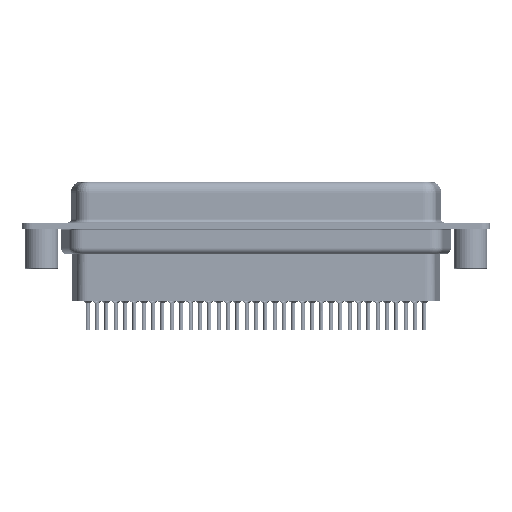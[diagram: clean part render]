
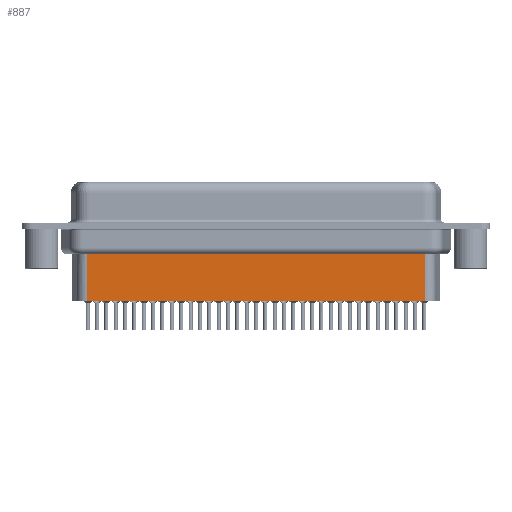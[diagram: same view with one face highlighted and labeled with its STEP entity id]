
A CAD part, front view. The second image highlights one B-rep face of the part: STEP entity #887.
In plain terms, the highlighted planar face has unit normal (0, -1, 0).
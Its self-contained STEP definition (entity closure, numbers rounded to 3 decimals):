
#887 = ADVANCED_FACE ( 'NONE', ( #9429 ), #2187, .T. ) ;
#2187 = PLANE ( 'NONE',  #17542 ) ;
#3297 = EDGE_CURVE ( 'NONE', #29896, #18458, #24506, .T. ) ;
#3354 = ORIENTED_EDGE ( 'NONE', *, *, #29043, .F. ) ;
#4019 = LINE ( 'NONE', #24741, #19696 ) ;
#4256 = ORIENTED_EDGE ( 'NONE', *, *, #20402, .F. ) ;
#4476 = DIRECTION ( 'NONE',  ( 0., 0., -1. ) ) ;
#6446 = CARTESIAN_POINT ( 'NONE',  ( 56.794, -3.5, -11.15 ) ) ;
#9429 = FACE_OUTER_BOUND ( 'NONE', #20702, .T. ) ;
#9587 = DIRECTION ( 'NONE',  ( -1., 0., 0. ) ) ;
#11562 = VECTOR ( 'NONE', #18019, 1000. ) ;
#11949 = DIRECTION ( 'NONE',  ( 0., -1., 0. ) ) ;
#13086 = CARTESIAN_POINT ( 'NONE',  ( 6.706, -3.5, -3.1 ) ) ;
#14567 = LINE ( 'NONE', #24340, #27772 ) ;
#15309 = ORIENTED_EDGE ( 'NONE', *, *, #3297, .T. ) ;
#17542 = AXIS2_PLACEMENT_3D ( 'NONE', #27446, #11949, #24753 ) ;
#18019 = DIRECTION ( 'NONE',  ( 0., 0., -1. ) ) ;
#18162 = VERTEX_POINT ( 'NONE', #6446 ) ;
#18458 = VERTEX_POINT ( 'NONE', #32302 ) ;
#19696 = VECTOR ( 'NONE', #9587, 1000. ) ;
#19812 = CARTESIAN_POINT ( 'NONE',  ( 6.459, -3.5, -4.097 ) ) ;
#20402 = EDGE_CURVE ( 'NONE', #18162, #31821, #4019, .T. ) ;
#20702 = EDGE_LOOP ( 'NONE', ( #3354, #15309, #23346, #4256 ) ) ;
#21692 = CARTESIAN_POINT ( 'NONE',  ( 6.706, -3.5, -11.15 ) ) ;
#21996 = VECTOR ( 'NONE', #32589, 1000. ) ;
#23346 = ORIENTED_EDGE ( 'NONE', *, *, #27051, .T. ) ;
#24340 = CARTESIAN_POINT ( 'NONE',  ( 56.794, -3.5, -3.1 ) ) ;
#24506 = LINE ( 'NONE', #19812, #21996 ) ;
#24741 = CARTESIAN_POINT ( 'NONE',  ( 6.706, -3.5, -11.15 ) ) ;
#24753 = DIRECTION ( 'NONE',  ( 1., 0., 0. ) ) ;
#27051 = EDGE_CURVE ( 'NONE', #18458, #31821, #29649, .T. ) ;
#27446 = CARTESIAN_POINT ( 'NONE',  ( 6.706, -3.5, -3.1 ) ) ;
#27772 = VECTOR ( 'NONE', #4476, 1000. ) ;
#29043 = EDGE_CURVE ( 'NONE', #29896, #18162, #14567, .T. ) ;
#29649 = LINE ( 'NONE', #13086, #11562 ) ;
#29896 = VERTEX_POINT ( 'NONE', #32346 ) ;
#31821 = VERTEX_POINT ( 'NONE', #21692 ) ;
#32302 = CARTESIAN_POINT ( 'NONE',  ( 6.706, -3.5, -4.097 ) ) ;
#32346 = CARTESIAN_POINT ( 'NONE',  ( 56.794, -3.5, -4.097 ) ) ;
#32589 = DIRECTION ( 'NONE',  ( -1., 0., 0. ) ) ;
